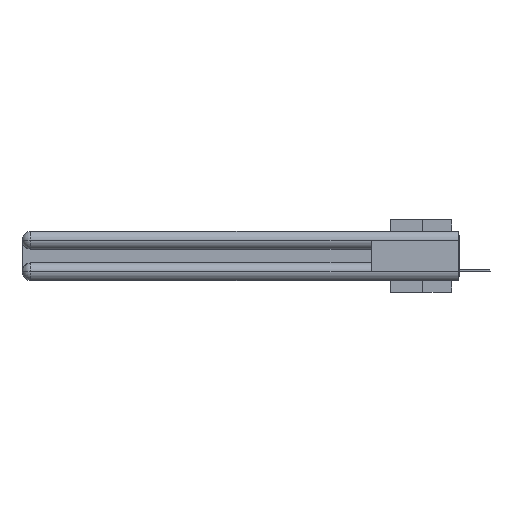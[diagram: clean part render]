
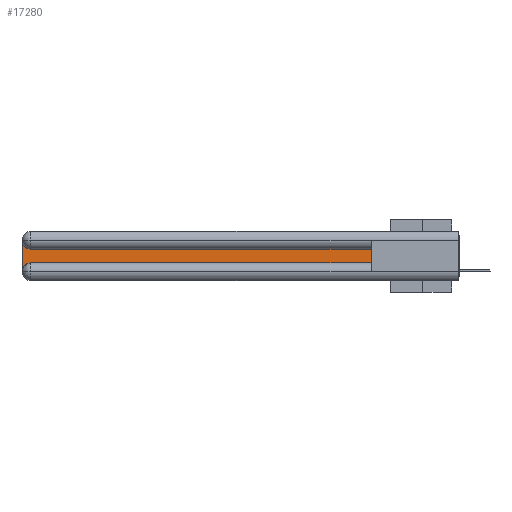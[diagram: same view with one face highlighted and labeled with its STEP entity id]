
A CAD part, left-side view. The second image highlights one B-rep face of the part: STEP entity #17280.
In plain terms, the highlighted planar face has unit normal (-1, 0, 0).
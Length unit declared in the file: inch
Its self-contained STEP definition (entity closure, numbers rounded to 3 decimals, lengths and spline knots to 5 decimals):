
#418 = VERTEX_POINT ( 'NONE', #20482 ) ;
#1633 = CARTESIAN_POINT ( 'NONE',  ( 0.075, 3., -0.2775 ) ) ;
#2219 = EDGE_CURVE ( 'NONE', #18675, #32567, #23931, .T. ) ;
#2376 = CARTESIAN_POINT ( 'NONE',  ( 0.075, 2.94, -0.2775 ) ) ;
#2495 = DIRECTION ( 'NONE',  ( 0., 0., -1. ) ) ;
#2639 = AXIS2_PLACEMENT_3D ( 'NONE', #22666, #31648, #2495 ) ;
#2806 = ORIENTED_EDGE ( 'NONE', *, *, #30083, .T. ) ;
#3448 = DIRECTION ( 'NONE',  ( 0., 0., -1. ) ) ;
#4836 = VERTEX_POINT ( 'NONE', #25725 ) ;
#4904 = CARTESIAN_POINT ( 'NONE',  ( 0.075, 0.6, -0.1225 ) ) ;
#5893 = DIRECTION ( 'NONE',  ( 0., 1., 0. ) ) ;
#6669 = CARTESIAN_POINT ( 'NONE',  ( 0.075, 3., -0.2175 ) ) ;
#8757 = DIRECTION ( 'NONE',  ( 1., 0., 0. ) ) ;
#9705 = VECTOR ( 'NONE', #36319, 39.37008 ) ;
#11698 = FACE_OUTER_BOUND ( 'NONE', #34902, .T. ) ;
#11761 = LINE ( 'NONE', #32692, #20439 ) ;
#12852 = DIRECTION ( 'NONE',  ( 0., 0., -1. ) ) ;
#14292 = DIRECTION ( 'NONE',  ( 1., 0., 0. ) ) ;
#14505 = CIRCLE ( 'NONE', #2639, 0.06 ) ;
#15130 = AXIS2_PLACEMENT_3D ( 'NONE', #2376, #14292, #3448 ) ;
#15665 = DIRECTION ( 'NONE',  ( 0., 0., -1. ) ) ;
#15911 = ORIENTED_EDGE ( 'NONE', *, *, #37824, .T. ) ;
#16083 = CARTESIAN_POINT ( 'NONE',  ( 0.075, 2.94, -0.2175 ) ) ;
#16429 = VERTEX_POINT ( 'NONE', #16083 ) ;
#16521 = AXIS2_PLACEMENT_3D ( 'NONE', #35543, #8757, #12852 ) ;
#17280 = ADVANCED_FACE ( 'NONE', ( #11698 ), #23661, .F. ) ;
#18675 = VERTEX_POINT ( 'NONE', #18725 ) ;
#18725 = CARTESIAN_POINT ( 'NONE',  ( 0.075, 3., -0.0625 ) ) ;
#19776 = VECTOR ( 'NONE', #32994, 39.37008 ) ;
#20439 = VECTOR ( 'NONE', #5893, 39.37008 ) ;
#20482 = CARTESIAN_POINT ( 'NONE',  ( 0.075, 0.6, -0.2175 ) ) ;
#20769 = EDGE_CURVE ( 'NONE', #33036, #4836, #11761, .T. ) ;
#21089 = LINE ( 'NONE', #26935, #19776 ) ;
#22666 = CARTESIAN_POINT ( 'NONE',  ( 0.075, 2.94, -0.0625 ) ) ;
#23127 = ORIENTED_EDGE ( 'NONE', *, *, #36195, .T. ) ;
#23661 = PLANE ( 'NONE',  #16521 ) ;
#23931 = LINE ( 'NONE', #6669, #30300 ) ;
#25725 = CARTESIAN_POINT ( 'NONE',  ( 0.075, 2.94, -0.1225 ) ) ;
#26935 = CARTESIAN_POINT ( 'NONE',  ( 0.075, 0.6, -0.2175 ) ) ;
#29365 = ORIENTED_EDGE ( 'NONE', *, *, #30550, .T. ) ;
#30083 = EDGE_CURVE ( 'NONE', #418, #33036, #30291, .T. ) ;
#30291 = LINE ( 'NONE', #32846, #9705 ) ;
#30300 = VECTOR ( 'NONE', #15665, 39.37008 ) ;
#30550 = EDGE_CURVE ( 'NONE', #16429, #418, #21089, .T. ) ;
#30636 = ORIENTED_EDGE ( 'NONE', *, *, #2219, .T. ) ;
#31648 = DIRECTION ( 'NONE',  ( 1., 0., 0. ) ) ;
#32567 = VERTEX_POINT ( 'NONE', #1633 ) ;
#32692 = CARTESIAN_POINT ( 'NONE',  ( 0.075, 0.6, -0.1225 ) ) ;
#32846 = CARTESIAN_POINT ( 'NONE',  ( 0.075, 0.6, -0.2175 ) ) ;
#32994 = DIRECTION ( 'NONE',  ( 0., -1., 0. ) ) ;
#33036 = VERTEX_POINT ( 'NONE', #4904 ) ;
#34902 = EDGE_LOOP ( 'NONE', ( #36749, #23127, #30636, #15911, #29365, #2806 ) ) ;
#35543 = CARTESIAN_POINT ( 'NONE',  ( 0.075, 3., -0.1225 ) ) ;
#36195 = EDGE_CURVE ( 'NONE', #4836, #18675, #14505, .T. ) ;
#36319 = DIRECTION ( 'NONE',  ( 0., 0., 1. ) ) ;
#36749 = ORIENTED_EDGE ( 'NONE', *, *, #20769, .T. ) ;
#36973 = CIRCLE ( 'NONE', #15130, 0.06 ) ;
#37824 = EDGE_CURVE ( 'NONE', #32567, #16429, #36973, .T. ) ;
